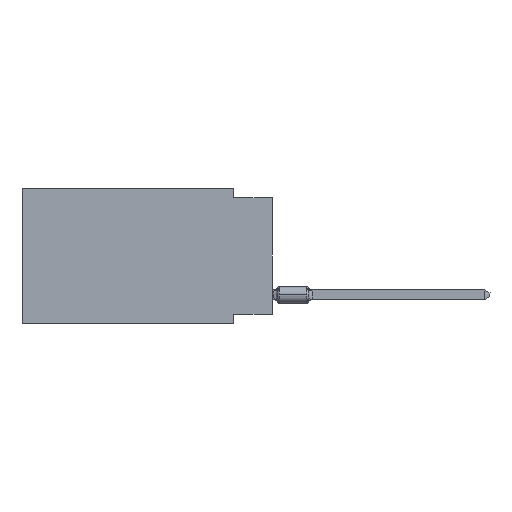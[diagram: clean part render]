
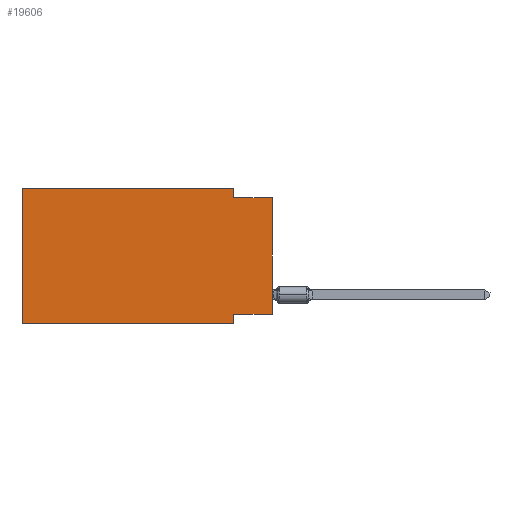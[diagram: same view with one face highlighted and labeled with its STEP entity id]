
A CAD part, left-side view. The second image highlights one B-rep face of the part: STEP entity #19606.
In plain terms, the highlighted planar face has unit normal (-1, 0, 0).
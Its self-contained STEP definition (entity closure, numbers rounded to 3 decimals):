
#220 = ORIENTED_EDGE ( 'NONE', *, *, #18103, .T. ) ;
#409 = ORIENTED_EDGE ( 'NONE', *, *, #3618, .T. ) ;
#1456 = ORIENTED_EDGE ( 'NONE', *, *, #20927, .F. ) ;
#2778 = CARTESIAN_POINT ( 'NONE',  ( 0., 16.383, 0. ) ) ;
#2980 = DIRECTION ( 'NONE',  ( 1., 0., 0. ) ) ;
#3127 = CARTESIAN_POINT ( 'NONE',  ( 0., 2.54, 0. ) ) ;
#3410 = VECTOR ( 'NONE', #6107, 1000. ) ;
#3618 = EDGE_CURVE ( 'NONE', #25086, #11774, #8003, .T. ) ;
#3785 = LINE ( 'NONE', #10179, #3410 ) ;
#4121 = EDGE_CURVE ( 'NONE', #15350, #20747, #19549, .T. ) ;
#4199 = DIRECTION ( 'NONE',  ( 0., -1., 0. ) ) ;
#4243 = CARTESIAN_POINT ( 'NONE',  ( 0., 0., -8.255 ) ) ;
#4432 = VERTEX_POINT ( 'NONE', #14454 ) ;
#4858 = ORIENTED_EDGE ( 'NONE', *, *, #21015, .F. ) ;
#5052 = VERTEX_POINT ( 'NONE', #22534 ) ;
#5203 = CARTESIAN_POINT ( 'NONE',  ( 0., 0., -0.635 ) ) ;
#5413 = FACE_OUTER_BOUND ( 'NONE', #12113, .T. ) ;
#5674 = LINE ( 'NONE', #7849, #23862 ) ;
#5990 = VECTOR ( 'NONE', #4199, 1000. ) ;
#6107 = DIRECTION ( 'NONE',  ( 0., 0., -1. ) ) ;
#7721 = PLANE ( 'NONE',  #14724 ) ;
#7849 = CARTESIAN_POINT ( 'NONE',  ( 0., 0., -0.635 ) ) ;
#7926 = ORIENTED_EDGE ( 'NONE', *, *, #17287, .F. ) ;
#8003 = LINE ( 'NONE', #16192, #20516 ) ;
#8762 = CARTESIAN_POINT ( 'NONE',  ( 0., 16.383, 0. ) ) ;
#8815 = CARTESIAN_POINT ( 'NONE',  ( 0., 2.54, 0. ) ) ;
#8903 = LINE ( 'NONE', #2778, #13777 ) ;
#9090 = CARTESIAN_POINT ( 'NONE',  ( 0., 16.383, -8.89 ) ) ;
#9250 = DIRECTION ( 'NONE',  ( 0., 0., -1. ) ) ;
#9371 = CARTESIAN_POINT ( 'NONE',  ( 0., 16.383, 0. ) ) ;
#9521 = VECTOR ( 'NONE', #13391, 1000. ) ;
#9717 = CARTESIAN_POINT ( 'NONE',  ( 0., 0., -8.255 ) ) ;
#10179 = CARTESIAN_POINT ( 'NONE',  ( 0., 2.54, -8.89 ) ) ;
#10576 = CARTESIAN_POINT ( 'NONE',  ( 0., 2.54, -8.89 ) ) ;
#11046 = ORIENTED_EDGE ( 'NONE', *, *, #4121, .F. ) ;
#11671 = DIRECTION ( 'NONE',  ( 0., -1., 0. ) ) ;
#11774 = VERTEX_POINT ( 'NONE', #5203 ) ;
#12113 = EDGE_LOOP ( 'NONE', ( #409, #18027, #4858, #11046, #7926, #220, #1456, #19778 ) ) ;
#12557 = DIRECTION ( 'NONE',  ( 0., 1., 0. ) ) ;
#12889 = LINE ( 'NONE', #8815, #20837 ) ;
#13391 = DIRECTION ( 'NONE',  ( 0., -1., 0. ) ) ;
#13548 = VERTEX_POINT ( 'NONE', #10576 ) ;
#13777 = VECTOR ( 'NONE', #25268, 1000. ) ;
#14454 = CARTESIAN_POINT ( 'NONE',  ( 0., 2.54, -0.635 ) ) ;
#14684 = LINE ( 'NONE', #24928, #5990 ) ;
#14724 = AXIS2_PLACEMENT_3D ( 'NONE', #9371, #2980, #9250 ) ;
#15350 = VERTEX_POINT ( 'NONE', #23928 ) ;
#16192 = CARTESIAN_POINT ( 'NONE',  ( 0., 0., 0. ) ) ;
#17287 = EDGE_CURVE ( 'NONE', #25738, #15350, #8903, .T. ) ;
#18027 = ORIENTED_EDGE ( 'NONE', *, *, #26346, .F. ) ;
#18103 = EDGE_CURVE ( 'NONE', #25738, #13548, #14684, .T. ) ;
#18912 = DIRECTION ( 'NONE',  ( 0., 0., -1. ) ) ;
#19549 = LINE ( 'NONE', #8762, #9521 ) ;
#19606 = ADVANCED_FACE ( 'NONE', ( #5413 ), #7721, .F. ) ;
#19778 = ORIENTED_EDGE ( 'NONE', *, *, #23463, .F. ) ;
#20516 = VECTOR ( 'NONE', #24381, 1000. ) ;
#20747 = VERTEX_POINT ( 'NONE', #3127 ) ;
#20837 = VECTOR ( 'NONE', #18912, 1000. ) ;
#20927 = EDGE_CURVE ( 'NONE', #5052, #13548, #3785, .T. ) ;
#21015 = EDGE_CURVE ( 'NONE', #20747, #4432, #12889, .T. ) ;
#22534 = CARTESIAN_POINT ( 'NONE',  ( 0., 2.54, -8.255 ) ) ;
#23463 = EDGE_CURVE ( 'NONE', #25086, #5052, #24694, .T. ) ;
#23862 = VECTOR ( 'NONE', #11671, 1000. ) ;
#23928 = CARTESIAN_POINT ( 'NONE',  ( 0., 16.383, 0. ) ) ;
#24381 = DIRECTION ( 'NONE',  ( 0., 0., 1. ) ) ;
#24694 = LINE ( 'NONE', #4243, #25085 ) ;
#24928 = CARTESIAN_POINT ( 'NONE',  ( 0., 16.383, -8.89 ) ) ;
#25085 = VECTOR ( 'NONE', #12557, 1000. ) ;
#25086 = VERTEX_POINT ( 'NONE', #9717 ) ;
#25268 = DIRECTION ( 'NONE',  ( 0., 0., 1. ) ) ;
#25738 = VERTEX_POINT ( 'NONE', #9090 ) ;
#26346 = EDGE_CURVE ( 'NONE', #4432, #11774, #5674, .T. ) ;
